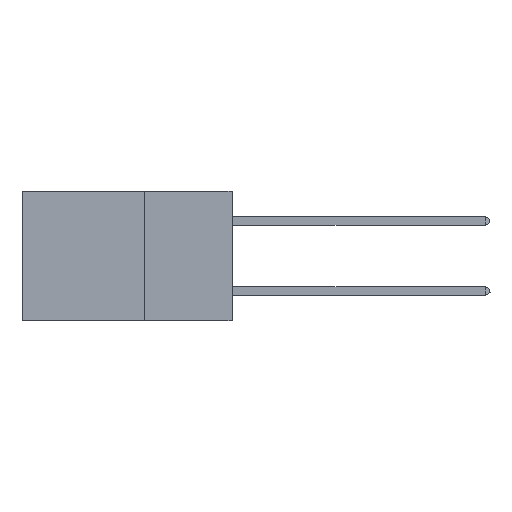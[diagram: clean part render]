
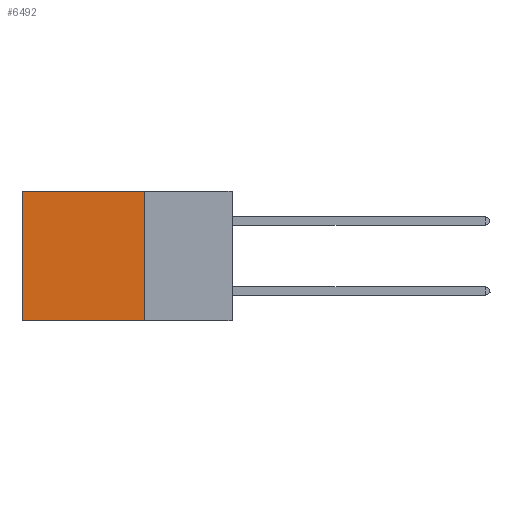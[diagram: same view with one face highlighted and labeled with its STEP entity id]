
A CAD part, left-side view. The second image highlights one B-rep face of the part: STEP entity #6492.
In plain terms, the highlighted planar face has unit normal (-1, 0, 0).
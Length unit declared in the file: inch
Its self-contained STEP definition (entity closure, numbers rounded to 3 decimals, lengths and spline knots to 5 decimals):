
#110 = VERTEX_POINT ( 'NONE', #3497 ) ;
#205 = VERTEX_POINT ( 'NONE', #9016 ) ;
#407 = DIRECTION ( 'NONE',  ( 0., 0., -1. ) ) ;
#456 = DIRECTION ( 'NONE',  ( 0., 0., -1. ) ) ;
#788 = CARTESIAN_POINT ( 'NONE',  ( 0.2875, 0.25, -0.37 ) ) ;
#1862 = LINE ( 'NONE', #8820, #2731 ) ;
#2731 = VECTOR ( 'NONE', #4241, 39.37008 ) ;
#2782 = ORIENTED_EDGE ( 'NONE', *, *, #3853, .F. ) ;
#2806 = EDGE_CURVE ( 'NONE', #205, #12355, #7691, .T. ) ;
#2903 = ORIENTED_EDGE ( 'NONE', *, *, #7850, .T. ) ;
#2937 = LINE ( 'NONE', #12845, #14246 ) ;
#3129 = ORIENTED_EDGE ( 'NONE', *, *, #2806, .F. ) ;
#3273 = EDGE_CURVE ( 'NONE', #3689, #110, #2937, .T. ) ;
#3497 = CARTESIAN_POINT ( 'NONE',  ( 0.2875, 0.6, -0.37 ) ) ;
#3689 = VERTEX_POINT ( 'NONE', #13707 ) ;
#3853 = EDGE_CURVE ( 'NONE', #12355, #110, #6626, .T. ) ;
#4241 = DIRECTION ( 'NONE',  ( 0., 1., 0. ) ) ;
#5250 = PLANE ( 'NONE',  #6455 ) ;
#5764 = VECTOR ( 'NONE', #407, 39.37008 ) ;
#6455 = AXIS2_PLACEMENT_3D ( 'NONE', #10267, #9609, #9208 ) ;
#6492 = ADVANCED_FACE ( 'NONE', ( #13893 ), #5250, .F. ) ;
#6626 = LINE ( 'NONE', #8501, #8911 ) ;
#7691 = LINE ( 'NONE', #12747, #5764 ) ;
#7850 = EDGE_CURVE ( 'NONE', #205, #3689, #1862, .T. ) ;
#8192 = EDGE_LOOP ( 'NONE', ( #13729, #2782, #3129, #2903 ) ) ;
#8501 = CARTESIAN_POINT ( 'NONE',  ( 0.2875, 0.25, -0.37 ) ) ;
#8820 = CARTESIAN_POINT ( 'NONE',  ( 0.2875, 0.25, 0. ) ) ;
#8911 = VECTOR ( 'NONE', #9610, 39.37008 ) ;
#9016 = CARTESIAN_POINT ( 'NONE',  ( 0.2875, 0.25, 0. ) ) ;
#9208 = DIRECTION ( 'NONE',  ( 0., 0., -1. ) ) ;
#9609 = DIRECTION ( 'NONE',  ( 1., 0., 0. ) ) ;
#9610 = DIRECTION ( 'NONE',  ( 0., 1., 0. ) ) ;
#10267 = CARTESIAN_POINT ( 'NONE',  ( 0.2875, 0.25, 0. ) ) ;
#12355 = VERTEX_POINT ( 'NONE', #788 ) ;
#12747 = CARTESIAN_POINT ( 'NONE',  ( 0.2875, 0.25, 0. ) ) ;
#12845 = CARTESIAN_POINT ( 'NONE',  ( 0.2875, 0.6, 0. ) ) ;
#13707 = CARTESIAN_POINT ( 'NONE',  ( 0.2875, 0.6, 0. ) ) ;
#13729 = ORIENTED_EDGE ( 'NONE', *, *, #3273, .T. ) ;
#13893 = FACE_OUTER_BOUND ( 'NONE', #8192, .T. ) ;
#14246 = VECTOR ( 'NONE', #456, 39.37008 ) ;
